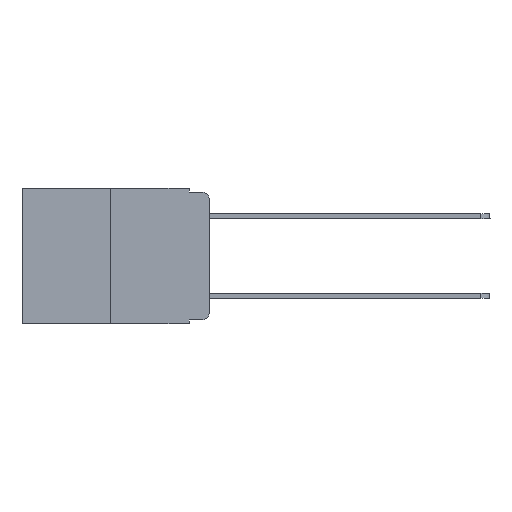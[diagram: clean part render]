
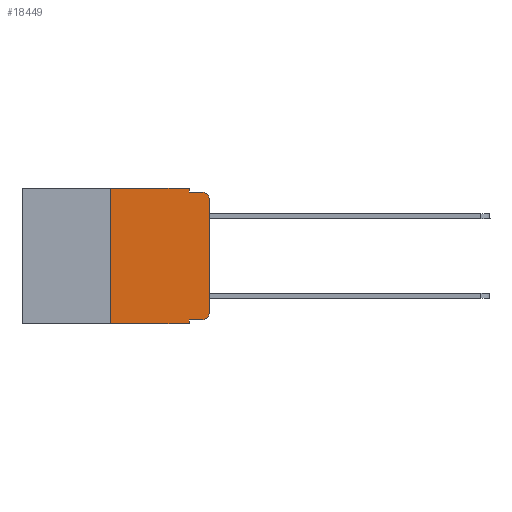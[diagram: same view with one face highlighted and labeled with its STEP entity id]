
A CAD part, left-side view. The second image highlights one B-rep face of the part: STEP entity #18449.
In plain terms, the highlighted planar face has unit normal (-1, 0, 0).
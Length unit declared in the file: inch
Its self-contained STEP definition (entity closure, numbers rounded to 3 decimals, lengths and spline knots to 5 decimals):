
#7 = VERTEX_POINT ( 'NONE', #7894 ) ;
#185 = VERTEX_POINT ( 'NONE', #17856 ) ;
#224 = CARTESIAN_POINT ( 'NONE',  ( 0., 0.051, -0.01 ) ) ;
#457 = CARTESIAN_POINT ( 'NONE',  ( 0., 0.473, 0. ) ) ;
#740 = EDGE_CURVE ( 'NONE', #7, #901, #6095, .T. ) ;
#901 = VERTEX_POINT ( 'NONE', #3718 ) ;
#1057 = EDGE_CURVE ( 'NONE', #185, #5002, #1428, .T. ) ;
#1226 = DIRECTION ( 'NONE',  ( 0., -1., 0. ) ) ;
#1428 = CIRCLE ( 'NONE', #7037, 0.02 ) ;
#1492 = DIRECTION ( 'NONE',  ( 0., 0., -1. ) ) ;
#1640 = VERTEX_POINT ( 'NONE', #6219 ) ;
#1733 = EDGE_CURVE ( 'NONE', #5002, #7, #6113, .T. ) ;
#2431 = EDGE_CURVE ( 'NONE', #13653, #6154, #6939, .T. ) ;
#2567 = DIRECTION ( 'NONE',  ( 0., -1., 0. ) ) ;
#2572 = ORIENTED_EDGE ( 'NONE', *, *, #12231, .T. ) ;
#2899 = ORIENTED_EDGE ( 'NONE', *, *, #14907, .F. ) ;
#3079 = DIRECTION ( 'NONE',  ( 1., 0., 0. ) ) ;
#3473 = AXIS2_PLACEMENT_3D ( 'NONE', #457, #3079, #15316 ) ;
#3476 = FACE_OUTER_BOUND ( 'NONE', #4452, .T. ) ;
#3505 = VERTEX_POINT ( 'NONE', #5903 ) ;
#3650 = EDGE_CURVE ( 'NONE', #6154, #901, #18467, .T. ) ;
#3679 = VECTOR ( 'NONE', #1226, 39.37008 ) ;
#3718 = CARTESIAN_POINT ( 'NONE',  ( 0., 0.02, -0.01 ) ) ;
#4002 = CARTESIAN_POINT ( 'NONE',  ( 0., 0.051, 0. ) ) ;
#4329 = VECTOR ( 'NONE', #11932, 39.37008 ) ;
#4452 = EDGE_LOOP ( 'NONE', ( #11026, #9470, #6829, #8975, #2899, #7001, #6445, #7589, #2572, #16555 ) ) ;
#4791 = DIRECTION ( 'NONE',  ( -1., 0., 0. ) ) ;
#5002 = VERTEX_POINT ( 'NONE', #13368 ) ;
#5007 = VECTOR ( 'NONE', #5497, 39.37008 ) ;
#5497 = DIRECTION ( 'NONE',  ( 0., -1., 0. ) ) ;
#5755 = DIRECTION ( 'NONE',  ( -1., 0., 0. ) ) ;
#5811 = CARTESIAN_POINT ( 'NONE',  ( 0., 0.25, -0.343 ) ) ;
#5903 = CARTESIAN_POINT ( 'NONE',  ( 0., 0.051, -0.343 ) ) ;
#5928 = LINE ( 'NONE', #10325, #4329 ) ;
#6095 = CIRCLE ( 'NONE', #7026, 0.02 ) ;
#6113 = LINE ( 'NONE', #7680, #15818 ) ;
#6154 = VERTEX_POINT ( 'NONE', #224 ) ;
#6219 = CARTESIAN_POINT ( 'NONE',  ( 0., 0.25, 0. ) ) ;
#6445 = ORIENTED_EDGE ( 'NONE', *, *, #9721, .T. ) ;
#6829 = ORIENTED_EDGE ( 'NONE', *, *, #3650, .F. ) ;
#6901 = DIRECTION ( 'NONE',  ( 0., 0., 1. ) ) ;
#6939 = LINE ( 'NONE', #4002, #13991 ) ;
#7001 = ORIENTED_EDGE ( 'NONE', *, *, #16835, .F. ) ;
#7026 = AXIS2_PLACEMENT_3D ( 'NONE', #9294, #4791, #1492 ) ;
#7037 = AXIS2_PLACEMENT_3D ( 'NONE', #16145, #5755, #14668 ) ;
#7112 = LINE ( 'NONE', #13110, #18573 ) ;
#7456 = VECTOR ( 'NONE', #6901, 39.37008 ) ;
#7589 = ORIENTED_EDGE ( 'NONE', *, *, #18763, .F. ) ;
#7680 = CARTESIAN_POINT ( 'NONE',  ( 0., 0., 0. ) ) ;
#7870 = PLANE ( 'NONE',  #3473 ) ;
#7894 = CARTESIAN_POINT ( 'NONE',  ( 0., 0., -0.03 ) ) ;
#8975 = ORIENTED_EDGE ( 'NONE', *, *, #2431, .F. ) ;
#9294 = CARTESIAN_POINT ( 'NONE',  ( 0., 0.02, -0.03 ) ) ;
#9470 = ORIENTED_EDGE ( 'NONE', *, *, #740, .T. ) ;
#9721 = EDGE_CURVE ( 'NONE', #17001, #3505, #5928, .T. ) ;
#10085 = CARTESIAN_POINT ( 'NONE',  ( 0., 0.051, -0.01 ) ) ;
#10277 = CARTESIAN_POINT ( 'NONE',  ( 0., 0.051, 0. ) ) ;
#10325 = CARTESIAN_POINT ( 'NONE',  ( 0., 0.473, -0.343 ) ) ;
#11026 = ORIENTED_EDGE ( 'NONE', *, *, #1733, .T. ) ;
#11693 = LINE ( 'NONE', #10277, #17497 ) ;
#11932 = DIRECTION ( 'NONE',  ( 0., -1., 0. ) ) ;
#12231 = EDGE_CURVE ( 'NONE', #13643, #185, #7112, .T. ) ;
#13110 = CARTESIAN_POINT ( 'NONE',  ( 0., 0.051, -0.333 ) ) ;
#13154 = DIRECTION ( 'NONE',  ( 0., 0., -1. ) ) ;
#13168 = CARTESIAN_POINT ( 'NONE',  ( 0., 0.473, 0. ) ) ;
#13368 = CARTESIAN_POINT ( 'NONE',  ( 0., 0., -0.313 ) ) ;
#13643 = VERTEX_POINT ( 'NONE', #15116 ) ;
#13653 = VERTEX_POINT ( 'NONE', #17959 ) ;
#13656 = DIRECTION ( 'NONE',  ( 0., 0., 1. ) ) ;
#13991 = VECTOR ( 'NONE', #14771, 39.37008 ) ;
#14616 = LINE ( 'NONE', #13168, #3679 ) ;
#14668 = DIRECTION ( 'NONE',  ( 0., 0., -1. ) ) ;
#14771 = DIRECTION ( 'NONE',  ( 0., 0., -1. ) ) ;
#14907 = EDGE_CURVE ( 'NONE', #1640, #13653, #14616, .T. ) ;
#15116 = CARTESIAN_POINT ( 'NONE',  ( 0., 0.051, -0.333 ) ) ;
#15316 = DIRECTION ( 'NONE',  ( 0., 0., -1. ) ) ;
#15818 = VECTOR ( 'NONE', #13656, 39.37008 ) ;
#16145 = CARTESIAN_POINT ( 'NONE',  ( 0., 0.02, -0.313 ) ) ;
#16555 = ORIENTED_EDGE ( 'NONE', *, *, #1057, .T. ) ;
#16835 = EDGE_CURVE ( 'NONE', #17001, #1640, #18791, .T. ) ;
#17001 = VERTEX_POINT ( 'NONE', #5811 ) ;
#17385 = CARTESIAN_POINT ( 'NONE',  ( 0., 0.25, 0. ) ) ;
#17497 = VECTOR ( 'NONE', #13154, 39.37008 ) ;
#17856 = CARTESIAN_POINT ( 'NONE',  ( 0., 0.02, -0.333 ) ) ;
#17959 = CARTESIAN_POINT ( 'NONE',  ( 0., 0.051, 0. ) ) ;
#18449 = ADVANCED_FACE ( 'NONE', ( #3476 ), #7870, .F. ) ;
#18467 = LINE ( 'NONE', #10085, #5007 ) ;
#18573 = VECTOR ( 'NONE', #2567, 39.37008 ) ;
#18763 = EDGE_CURVE ( 'NONE', #13643, #3505, #11693, .T. ) ;
#18791 = LINE ( 'NONE', #17385, #7456 ) ;
